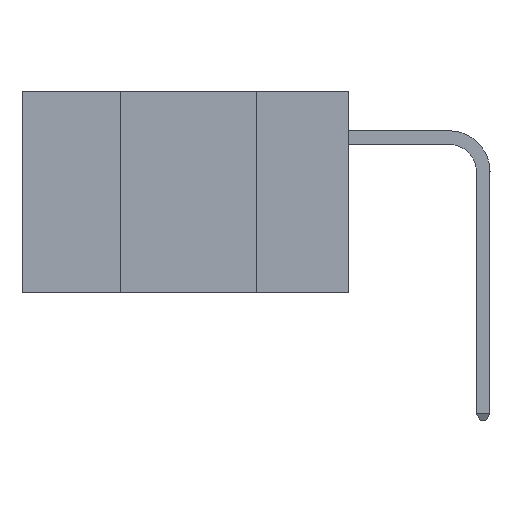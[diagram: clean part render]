
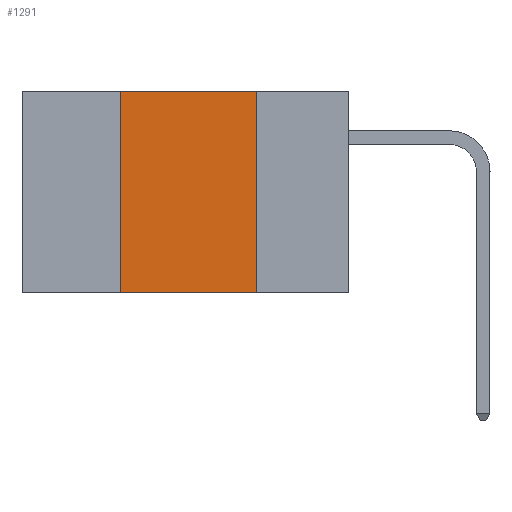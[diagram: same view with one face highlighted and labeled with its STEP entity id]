
A CAD part, left-side view. The second image highlights one B-rep face of the part: STEP entity #1291.
In plain terms, the highlighted planar face has unit normal (-1, 0, 0).
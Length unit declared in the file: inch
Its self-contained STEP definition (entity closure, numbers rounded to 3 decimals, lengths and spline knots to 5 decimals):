
#85 = EDGE_CURVE ( 'NONE', #20027, #3446, #13301, .T. ) ;
#210 = CARTESIAN_POINT ( 'NONE',  ( 0., 0.6, 0. ) ) ;
#714 = EDGE_CURVE ( 'NONE', #20054, #14668, #12430, .T. ) ;
#1291 = ADVANCED_FACE ( 'NONE', ( #13822 ), #15607, .F. ) ;
#1677 = ORIENTED_EDGE ( 'NONE', *, *, #85, .T. ) ;
#2012 = CARTESIAN_POINT ( 'NONE',  ( 0., 0.42, 0. ) ) ;
#2493 = VECTOR ( 'NONE', #17509, 39.37008 ) ;
#2916 = VECTOR ( 'NONE', #9376, 39.37008 ) ;
#3446 = VERTEX_POINT ( 'NONE', #15461 ) ;
#3641 = ORIENTED_EDGE ( 'NONE', *, *, #714, .F. ) ;
#3821 = DIRECTION ( 'NONE',  ( 0., 0., 1. ) ) ;
#4033 = CARTESIAN_POINT ( 'NONE',  ( 0., 0.17, 0. ) ) ;
#4941 = CARTESIAN_POINT ( 'NONE',  ( 0., 0.17, 0. ) ) ;
#5474 = EDGE_CURVE ( 'NONE', #20027, #20054, #14666, .T. ) ;
#7365 = VECTOR ( 'NONE', #9871, 39.37008 ) ;
#9376 = DIRECTION ( 'NONE',  ( 0., -1., 0. ) ) ;
#9835 = VECTOR ( 'NONE', #3821, 39.37008 ) ;
#9871 = DIRECTION ( 'NONE',  ( 0., -1., 0. ) ) ;
#12430 = LINE ( 'NONE', #210, #2916 ) ;
#13301 = LINE ( 'NONE', #17403, #7365 ) ;
#13822 = FACE_OUTER_BOUND ( 'NONE', #20316, .T. ) ;
#14666 = LINE ( 'NONE', #2012, #9835 ) ;
#14668 = VERTEX_POINT ( 'NONE', #4033 ) ;
#15378 = CARTESIAN_POINT ( 'NONE',  ( 0., 0.42, -0.37 ) ) ;
#15461 = CARTESIAN_POINT ( 'NONE',  ( 0., 0.17, -0.37 ) ) ;
#15607 = PLANE ( 'NONE',  #22030 ) ;
#16228 = LINE ( 'NONE', #4941, #2493 ) ;
#16316 = CARTESIAN_POINT ( 'NONE',  ( 0., 0.6, 0. ) ) ;
#17256 = EDGE_CURVE ( 'NONE', #14668, #3446, #16228, .T. ) ;
#17301 = CARTESIAN_POINT ( 'NONE',  ( 0., 0.42, 0. ) ) ;
#17403 = CARTESIAN_POINT ( 'NONE',  ( 0., 0.6, -0.37 ) ) ;
#17407 = ORIENTED_EDGE ( 'NONE', *, *, #5474, .F. ) ;
#17509 = DIRECTION ( 'NONE',  ( 0., 0., -1. ) ) ;
#18551 = DIRECTION ( 'NONE',  ( 1., 0., 0. ) ) ;
#19919 = DIRECTION ( 'NONE',  ( 0., 0., -1. ) ) ;
#20027 = VERTEX_POINT ( 'NONE', #15378 ) ;
#20054 = VERTEX_POINT ( 'NONE', #17301 ) ;
#20316 = EDGE_LOOP ( 'NONE', ( #22943, #3641, #17407, #1677 ) ) ;
#22030 = AXIS2_PLACEMENT_3D ( 'NONE', #16316, #18551, #19919 ) ;
#22943 = ORIENTED_EDGE ( 'NONE', *, *, #17256, .F. ) ;
